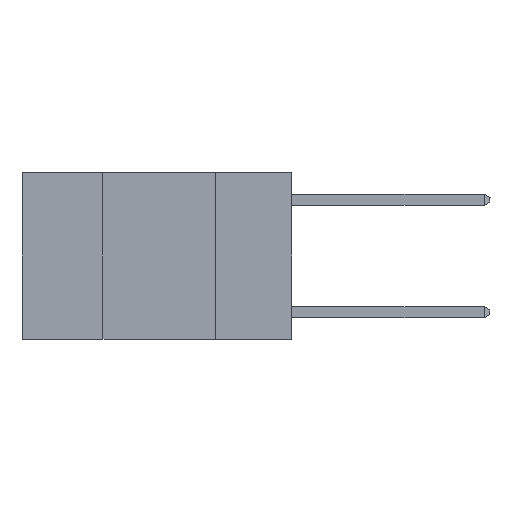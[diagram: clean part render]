
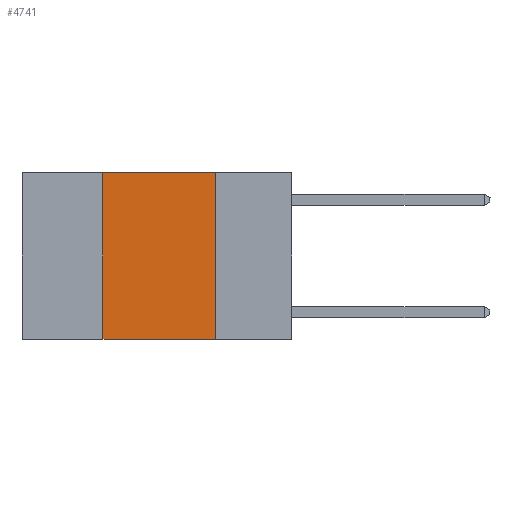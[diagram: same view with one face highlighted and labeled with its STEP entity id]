
A CAD part, left-side view. The second image highlights one B-rep face of the part: STEP entity #4741.
In plain terms, the highlighted planar face has unit normal (-1, 0, 0).
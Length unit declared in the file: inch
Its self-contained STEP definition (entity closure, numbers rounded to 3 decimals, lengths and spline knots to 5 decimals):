
#130 = EDGE_CURVE ( 'NONE', #4613, #8573, #3856, .T. ) ;
#152 = AXIS2_PLACEMENT_3D ( 'NONE', #475, #3214, #7896 ) ;
#313 = DIRECTION ( 'NONE',  ( 0., -1., 0. ) ) ;
#475 = CARTESIAN_POINT ( 'NONE',  ( 0., 0.6, 0. ) ) ;
#1032 = CARTESIAN_POINT ( 'NONE',  ( 0., 0.42, 0. ) ) ;
#1459 = ORIENTED_EDGE ( 'NONE', *, *, #2584, .F. ) ;
#2038 = EDGE_CURVE ( 'NONE', #3812, #3385, #2772, .T. ) ;
#2338 = DIRECTION ( 'NONE',  ( 0., -1., 0. ) ) ;
#2584 = EDGE_CURVE ( 'NONE', #3385, #4613, #6390, .T. ) ;
#2588 = FACE_OUTER_BOUND ( 'NONE', #4433, .T. ) ;
#2662 = VECTOR ( 'NONE', #313, 39.37008 ) ;
#2772 = LINE ( 'NONE', #8303, #3384 ) ;
#3214 = DIRECTION ( 'NONE',  ( 1., 0., 0. ) ) ;
#3384 = VECTOR ( 'NONE', #6770, 39.37008 ) ;
#3385 = VERTEX_POINT ( 'NONE', #1032 ) ;
#3812 = VERTEX_POINT ( 'NONE', #7782 ) ;
#3856 = LINE ( 'NONE', #4693, #8502 ) ;
#4406 = LINE ( 'NONE', #6422, #2662 ) ;
#4433 = EDGE_LOOP ( 'NONE', ( #7753, #1459, #7746, #8440 ) ) ;
#4613 = VERTEX_POINT ( 'NONE', #5651 ) ;
#4693 = CARTESIAN_POINT ( 'NONE',  ( 0., 0.17, 0. ) ) ;
#4741 = ADVANCED_FACE ( 'NONE', ( #2588 ), #8031, .F. ) ;
#5651 = CARTESIAN_POINT ( 'NONE',  ( 0., 0.17, 0. ) ) ;
#5711 = CARTESIAN_POINT ( 'NONE',  ( 0., 0.6, 0. ) ) ;
#6390 = LINE ( 'NONE', #5711, #7471 ) ;
#6422 = CARTESIAN_POINT ( 'NONE',  ( 0., 0.6, -0.37 ) ) ;
#6687 = DIRECTION ( 'NONE',  ( 0., 0., -1. ) ) ;
#6770 = DIRECTION ( 'NONE',  ( 0., 0., 1. ) ) ;
#7471 = VECTOR ( 'NONE', #2338, 39.37008 ) ;
#7746 = ORIENTED_EDGE ( 'NONE', *, *, #2038, .F. ) ;
#7753 = ORIENTED_EDGE ( 'NONE', *, *, #130, .F. ) ;
#7782 = CARTESIAN_POINT ( 'NONE',  ( 0., 0.42, -0.37 ) ) ;
#7896 = DIRECTION ( 'NONE',  ( 0., 0., -1. ) ) ;
#8031 = PLANE ( 'NONE',  #152 ) ;
#8182 = CARTESIAN_POINT ( 'NONE',  ( 0., 0.17, -0.37 ) ) ;
#8303 = CARTESIAN_POINT ( 'NONE',  ( 0., 0.42, 0. ) ) ;
#8431 = EDGE_CURVE ( 'NONE', #3812, #8573, #4406, .T. ) ;
#8440 = ORIENTED_EDGE ( 'NONE', *, *, #8431, .T. ) ;
#8502 = VECTOR ( 'NONE', #6687, 39.37008 ) ;
#8573 = VERTEX_POINT ( 'NONE', #8182 ) ;
